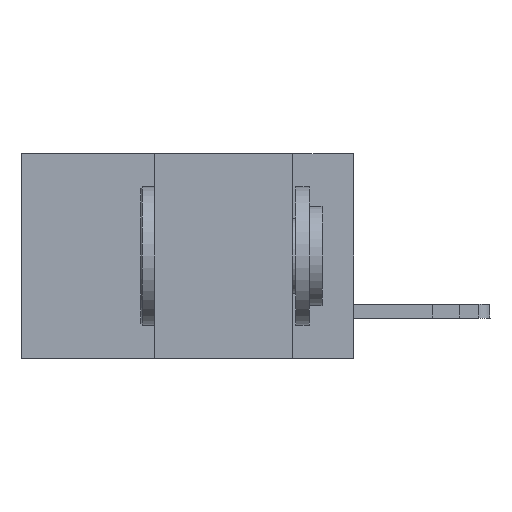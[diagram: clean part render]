
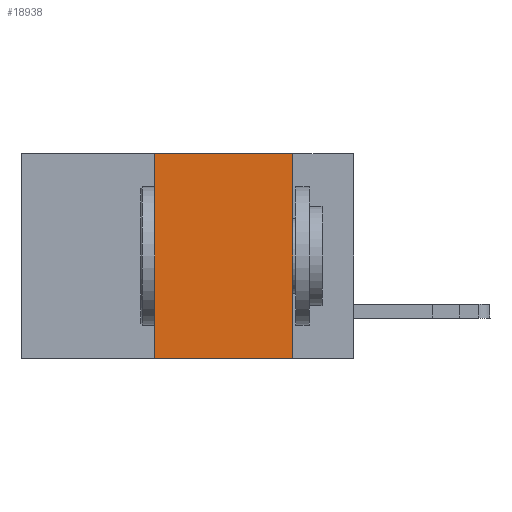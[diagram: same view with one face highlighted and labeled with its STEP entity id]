
A CAD part, left-side view. The second image highlights one B-rep face of the part: STEP entity #18938.
In plain terms, the highlighted planar face has unit normal (-1, 0, 0).
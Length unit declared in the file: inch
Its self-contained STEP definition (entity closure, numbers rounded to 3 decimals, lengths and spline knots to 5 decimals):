
#512 = LINE ( 'NONE', #18554, #23917 ) ;
#1429 = DIRECTION ( 'NONE',  ( 1., 0., 0. ) ) ;
#3478 = DIRECTION ( 'NONE',  ( 0., 0., -1. ) ) ;
#3566 = EDGE_CURVE ( 'NONE', #15414, #19794, #15398, .T. ) ;
#4811 = LINE ( 'NONE', #7991, #27725 ) ;
#5076 = CARTESIAN_POINT ( 'NONE',  ( 0., 0.36, 0. ) ) ;
#6188 = DIRECTION ( 'NONE',  ( 0., 0., -1. ) ) ;
#7234 = ORIENTED_EDGE ( 'NONE', *, *, #3566, .F. ) ;
#7872 = DIRECTION ( 'NONE',  ( 0., 0., 1. ) ) ;
#7991 = CARTESIAN_POINT ( 'NONE',  ( 0., 0.36, 0. ) ) ;
#8001 = ORIENTED_EDGE ( 'NONE', *, *, #27178, .F. ) ;
#9599 = CARTESIAN_POINT ( 'NONE',  ( 0., 0.6, 0. ) ) ;
#10284 = CARTESIAN_POINT ( 'NONE',  ( 0., 0.36, -0.37 ) ) ;
#10526 = LINE ( 'NONE', #21161, #30820 ) ;
#10651 = CARTESIAN_POINT ( 'NONE',  ( 0., 0.11, -0.37 ) ) ;
#11688 = CARTESIAN_POINT ( 'NONE',  ( 0., 0.11, 0. ) ) ;
#14372 = ORIENTED_EDGE ( 'NONE', *, *, #16772, .T. ) ;
#15363 = ORIENTED_EDGE ( 'NONE', *, *, #27331, .F. ) ;
#15398 = LINE ( 'NONE', #31004, #20770 ) ;
#15414 = VERTEX_POINT ( 'NONE', #5076 ) ;
#16772 = EDGE_CURVE ( 'NONE', #31693, #31196, #10526, .T. ) ;
#18232 = AXIS2_PLACEMENT_3D ( 'NONE', #9599, #1429, #3478 ) ;
#18554 = CARTESIAN_POINT ( 'NONE',  ( 0., 0.11, 0. ) ) ;
#18938 = ADVANCED_FACE ( 'NONE', ( #26377 ), #21798, .F. ) ;
#19794 = VERTEX_POINT ( 'NONE', #11688 ) ;
#20770 = VECTOR ( 'NONE', #23701, 39.37008 ) ;
#21096 = EDGE_LOOP ( 'NONE', ( #15363, #7234, #8001, #14372 ) ) ;
#21161 = CARTESIAN_POINT ( 'NONE',  ( 0., 0.6, -0.37 ) ) ;
#21798 = PLANE ( 'NONE',  #18232 ) ;
#23701 = DIRECTION ( 'NONE',  ( 0., -1., 0. ) ) ;
#23917 = VECTOR ( 'NONE', #6188, 39.37008 ) ;
#26377 = FACE_OUTER_BOUND ( 'NONE', #21096, .T. ) ;
#27178 = EDGE_CURVE ( 'NONE', #31693, #15414, #4811, .T. ) ;
#27331 = EDGE_CURVE ( 'NONE', #19794, #31196, #512, .T. ) ;
#27451 = DIRECTION ( 'NONE',  ( 0., -1., 0. ) ) ;
#27725 = VECTOR ( 'NONE', #7872, 39.37008 ) ;
#30820 = VECTOR ( 'NONE', #27451, 39.37008 ) ;
#31004 = CARTESIAN_POINT ( 'NONE',  ( 0., 0.6, 0. ) ) ;
#31196 = VERTEX_POINT ( 'NONE', #10651 ) ;
#31693 = VERTEX_POINT ( 'NONE', #10284 ) ;
